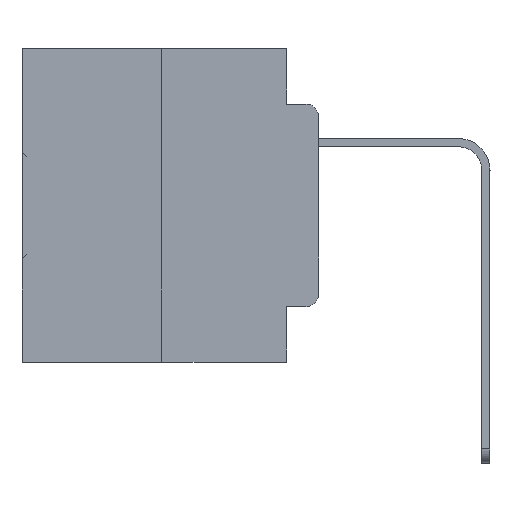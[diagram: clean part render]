
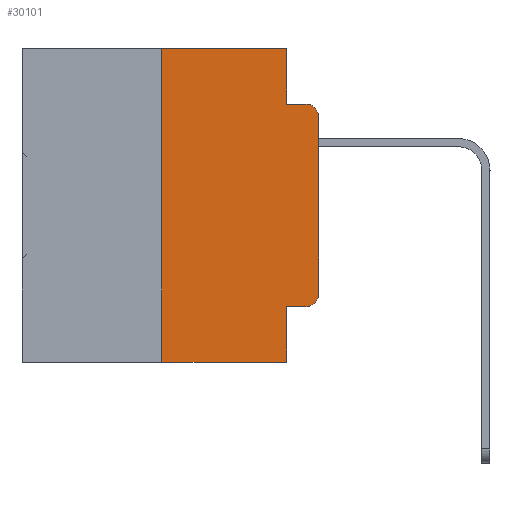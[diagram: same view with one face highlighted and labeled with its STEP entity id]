
A CAD part, left-side view. The second image highlights one B-rep face of the part: STEP entity #30101.
In plain terms, the highlighted planar face has unit normal (-1, 0, 0).
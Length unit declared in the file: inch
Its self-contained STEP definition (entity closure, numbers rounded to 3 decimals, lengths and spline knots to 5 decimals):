
#280 = DIRECTION ( 'NONE',  ( 0., -1., 0. ) ) ;
#311 = VECTOR ( 'NONE', #21311, 39.37008 ) ;
#576 = DIRECTION ( 'NONE',  ( 0., -1., 0. ) ) ;
#770 = VERTEX_POINT ( 'NONE', #32108 ) ;
#805 = ORIENTED_EDGE ( 'NONE', *, *, #10595, .F. ) ;
#858 = LINE ( 'NONE', #4593, #2927 ) ;
#892 = DIRECTION ( 'NONE',  ( -1., 0., 0. ) ) ;
#1023 = CARTESIAN_POINT ( 'NONE',  ( 0., 0.051, 0. ) ) ;
#1220 = DIRECTION ( 'NONE',  ( 0., 0., -1. ) ) ;
#1860 = CARTESIAN_POINT ( 'NONE',  ( 0., 0., -0.1085 ) ) ;
#2020 = DIRECTION ( 'NONE',  ( 0., 0., -1. ) ) ;
#2733 = VERTEX_POINT ( 'NONE', #10272 ) ;
#2742 = FACE_OUTER_BOUND ( 'NONE', #33768, .T. ) ;
#2927 = VECTOR ( 'NONE', #33385, 39.37008 ) ;
#3014 = CARTESIAN_POINT ( 'NONE',  ( 0., 0., 0. ) ) ;
#3330 = CARTESIAN_POINT ( 'NONE',  ( 0., 0.051, -0.0885 ) ) ;
#3416 = CARTESIAN_POINT ( 'NONE',  ( 0., 0.02, -0.4115 ) ) ;
#3864 = DIRECTION ( 'NONE',  ( 0., 0., -1. ) ) ;
#4092 = VERTEX_POINT ( 'NONE', #31221 ) ;
#4095 = CIRCLE ( 'NONE', #6029, 0.02 ) ;
#4593 = CARTESIAN_POINT ( 'NONE',  ( 0., 0.051, -0.0885 ) ) ;
#4657 = CARTESIAN_POINT ( 'NONE',  ( 0., 0.051, 0. ) ) ;
#4682 = LINE ( 'NONE', #13944, #11997 ) ;
#5315 = EDGE_CURVE ( 'NONE', #13901, #770, #4095, .T. ) ;
#5378 = CARTESIAN_POINT ( 'NONE',  ( 0., 0.051, 0. ) ) ;
#5950 = CARTESIAN_POINT ( 'NONE',  ( 0., 0.473, -0.5 ) ) ;
#6029 = AXIS2_PLACEMENT_3D ( 'NONE', #30122, #892, #3864 ) ;
#6957 = VERTEX_POINT ( 'NONE', #5378 ) ;
#7051 = LINE ( 'NONE', #31606, #14820 ) ;
#7298 = ORIENTED_EDGE ( 'NONE', *, *, #27623, .F. ) ;
#7906 = CARTESIAN_POINT ( 'NONE',  ( 0., 0.02, -0.0885 ) ) ;
#8316 = LINE ( 'NONE', #4657, #33279 ) ;
#9203 = PLANE ( 'NONE',  #30183 ) ;
#9628 = EDGE_CURVE ( 'NONE', #6957, #27256, #8316, .T. ) ;
#10147 = VERTEX_POINT ( 'NONE', #1860 ) ;
#10258 = CARTESIAN_POINT ( 'NONE',  ( 0., 0.25, 0. ) ) ;
#10272 = CARTESIAN_POINT ( 'NONE',  ( 0., 0.25, -0.5 ) ) ;
#10383 = CARTESIAN_POINT ( 'NONE',  ( 0., 0.051, -0.5 ) ) ;
#10595 = EDGE_CURVE ( 'NONE', #27256, #26310, #858, .T. ) ;
#11707 = CARTESIAN_POINT ( 'NONE',  ( 0., 0.473, 0. ) ) ;
#11997 = VECTOR ( 'NONE', #14398, 39.37008 ) ;
#12423 = LINE ( 'NONE', #10258, #25506 ) ;
#12795 = ORIENTED_EDGE ( 'NONE', *, *, #20169, .F. ) ;
#12854 = VECTOR ( 'NONE', #576, 39.37008 ) ;
#13901 = VERTEX_POINT ( 'NONE', #3416 ) ;
#13944 = CARTESIAN_POINT ( 'NONE',  ( 0., 0.473, 0. ) ) ;
#14398 = DIRECTION ( 'NONE',  ( 0., -1., 0. ) ) ;
#14820 = VECTOR ( 'NONE', #280, 39.37008 ) ;
#14835 = ORIENTED_EDGE ( 'NONE', *, *, #9628, .F. ) ;
#15126 = CARTESIAN_POINT ( 'NONE',  ( 0., 0.02, -0.1085 ) ) ;
#15911 = ORIENTED_EDGE ( 'NONE', *, *, #24476, .T. ) ;
#16564 = ORIENTED_EDGE ( 'NONE', *, *, #27223, .T. ) ;
#17381 = VERTEX_POINT ( 'NONE', #24598 ) ;
#19336 = DIRECTION ( 'NONE',  ( 0., 0., -1. ) ) ;
#20125 = CIRCLE ( 'NONE', #26335, 0.02 ) ;
#20169 = EDGE_CURVE ( 'NONE', #4092, #28781, #32193, .T. ) ;
#20443 = ORIENTED_EDGE ( 'NONE', *, *, #24766, .T. ) ;
#21311 = DIRECTION ( 'NONE',  ( 0., 0., 1. ) ) ;
#22008 = LINE ( 'NONE', #3014, #311 ) ;
#23481 = LINE ( 'NONE', #5950, #12854 ) ;
#24318 = ORIENTED_EDGE ( 'NONE', *, *, #27409, .F. ) ;
#24476 = EDGE_CURVE ( 'NONE', #4092, #13901, #7051, .T. ) ;
#24598 = CARTESIAN_POINT ( 'NONE',  ( 0., 0.25, 0. ) ) ;
#24766 = EDGE_CURVE ( 'NONE', #10147, #26310, #20125, .T. ) ;
#24960 = DIRECTION ( 'NONE',  ( 1., 0., 0. ) ) ;
#25219 = VECTOR ( 'NONE', #19336, 39.37008 ) ;
#25506 = VECTOR ( 'NONE', #28067, 39.37008 ) ;
#26310 = VERTEX_POINT ( 'NONE', #7906 ) ;
#26335 = AXIS2_PLACEMENT_3D ( 'NONE', #15126, #30553, #28122 ) ;
#27223 = EDGE_CURVE ( 'NONE', #2733, #28781, #23481, .T. ) ;
#27256 = VERTEX_POINT ( 'NONE', #3330 ) ;
#27409 = EDGE_CURVE ( 'NONE', #17381, #6957, #4682, .T. ) ;
#27623 = EDGE_CURVE ( 'NONE', #2733, #17381, #12423, .T. ) ;
#28067 = DIRECTION ( 'NONE',  ( 0., 0., 1. ) ) ;
#28122 = DIRECTION ( 'NONE',  ( 0., 0., -1. ) ) ;
#28359 = ORIENTED_EDGE ( 'NONE', *, *, #5315, .T. ) ;
#28781 = VERTEX_POINT ( 'NONE', #10383 ) ;
#30101 = ADVANCED_FACE ( 'NONE', ( #2742 ), #9203, .F. ) ;
#30122 = CARTESIAN_POINT ( 'NONE',  ( 0., 0.02, -0.3915 ) ) ;
#30183 = AXIS2_PLACEMENT_3D ( 'NONE', #11707, #24960, #1220 ) ;
#30540 = EDGE_CURVE ( 'NONE', #770, #10147, #22008, .T. ) ;
#30553 = DIRECTION ( 'NONE',  ( -1., 0., 0. ) ) ;
#31221 = CARTESIAN_POINT ( 'NONE',  ( 0., 0.051, -0.4115 ) ) ;
#31606 = CARTESIAN_POINT ( 'NONE',  ( 0., 0.051, -0.4115 ) ) ;
#32108 = CARTESIAN_POINT ( 'NONE',  ( 0., 0., -0.3915 ) ) ;
#32193 = LINE ( 'NONE', #1023, #25219 ) ;
#32589 = ORIENTED_EDGE ( 'NONE', *, *, #30540, .T. ) ;
#33279 = VECTOR ( 'NONE', #2020, 39.37008 ) ;
#33385 = DIRECTION ( 'NONE',  ( 0., -1., 0. ) ) ;
#33768 = EDGE_LOOP ( 'NONE', ( #32589, #20443, #805, #14835, #24318, #7298, #16564, #12795, #15911, #28359 ) ) ;
